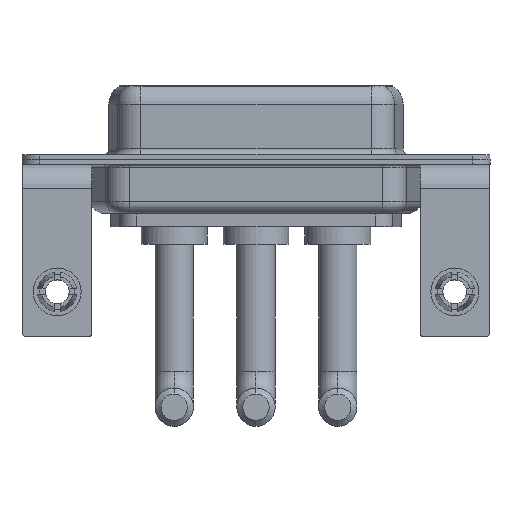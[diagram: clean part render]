
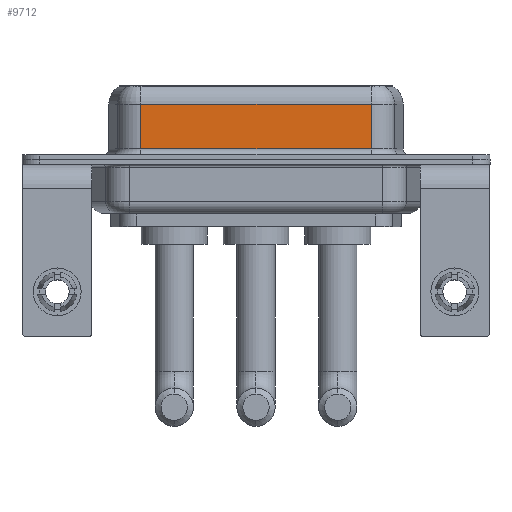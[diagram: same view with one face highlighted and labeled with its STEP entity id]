
A CAD part, front view. The second image highlights one B-rep face of the part: STEP entity #9712.
In plain terms, the highlighted planar face has unit normal (0, -1, 0).
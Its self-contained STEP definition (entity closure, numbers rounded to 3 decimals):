
#526 = DIRECTION ( 'NONE',  ( 0., 0., -1. ) ) ;
#994 = CARTESIAN_POINT ( 'NONE',  ( 26.287, -3.95, 0.9 ) ) ;
#1103 = VERTEX_POINT ( 'NONE', #13853 ) ;
#1294 = CARTESIAN_POINT ( 'NONE',  ( 26.287, -3.95, 4.65 ) ) ;
#2367 = EDGE_CURVE ( 'NONE', #3149, #6838, #10752, .T. ) ;
#3055 = VECTOR ( 'NONE', #14198, 1000. ) ;
#3149 = VERTEX_POINT ( 'NONE', #1294 ) ;
#4361 = LINE ( 'NONE', #10798, #12250 ) ;
#4734 = CARTESIAN_POINT ( 'NONE',  ( 7.013, -3.95, 6.4 ) ) ;
#4735 = DIRECTION ( 'NONE',  ( 0., 0., 1. ) ) ;
#5014 = CARTESIAN_POINT ( 'NONE',  ( 26.287, -3.95, 4.65 ) ) ;
#5320 = CARTESIAN_POINT ( 'NONE',  ( 7.013, -3.95, 0.9 ) ) ;
#5743 = ORIENTED_EDGE ( 'NONE', *, *, #9606, .F. ) ;
#6760 = AXIS2_PLACEMENT_3D ( 'NONE', #10392, #9047, #4735 ) ;
#6838 = VERTEX_POINT ( 'NONE', #7891 ) ;
#7387 = EDGE_CURVE ( 'NONE', #6838, #7709, #13615, .T. ) ;
#7709 = VERTEX_POINT ( 'NONE', #5320 ) ;
#7891 = CARTESIAN_POINT ( 'NONE',  ( 7.013, -3.95, 4.65 ) ) ;
#8165 = EDGE_LOOP ( 'NONE', ( #5743, #9603, #11492, #9319 ) ) ;
#9047 = DIRECTION ( 'NONE',  ( 0., 1., 0. ) ) ;
#9319 = ORIENTED_EDGE ( 'NONE', *, *, #10662, .T. ) ;
#9603 = ORIENTED_EDGE ( 'NONE', *, *, #2367, .T. ) ;
#9606 = EDGE_CURVE ( 'NONE', #3149, #1103, #4361, .T. ) ;
#9712 = ADVANCED_FACE ( 'NONE', ( #11440 ), #12569, .F. ) ;
#10392 = CARTESIAN_POINT ( 'NONE',  ( 26.287, -3.95, 6.4 ) ) ;
#10662 = EDGE_CURVE ( 'NONE', #7709, #1103, #11196, .T. ) ;
#10752 = LINE ( 'NONE', #5014, #3055 ) ;
#10798 = CARTESIAN_POINT ( 'NONE',  ( 26.287, -3.95, 6.4 ) ) ;
#11196 = LINE ( 'NONE', #994, #14422 ) ;
#11440 = FACE_OUTER_BOUND ( 'NONE', #8165, .T. ) ;
#11492 = ORIENTED_EDGE ( 'NONE', *, *, #7387, .T. ) ;
#12250 = VECTOR ( 'NONE', #526, 1000. ) ;
#12569 = PLANE ( 'NONE',  #6760 ) ;
#12714 = DIRECTION ( 'NONE',  ( 0., 0., -1. ) ) ;
#12893 = DIRECTION ( 'NONE',  ( 1., 0., 0. ) ) ;
#13615 = LINE ( 'NONE', #4734, #13861 ) ;
#13853 = CARTESIAN_POINT ( 'NONE',  ( 26.287, -3.95, 0.9 ) ) ;
#13861 = VECTOR ( 'NONE', #12714, 1000. ) ;
#14198 = DIRECTION ( 'NONE',  ( -1., 0., 0. ) ) ;
#14422 = VECTOR ( 'NONE', #12893, 1000. ) ;
